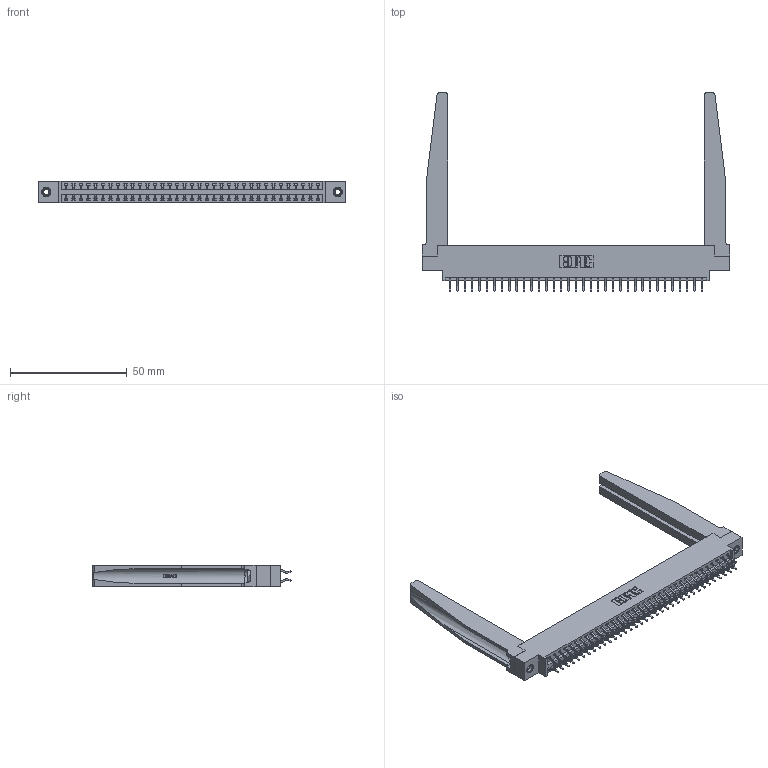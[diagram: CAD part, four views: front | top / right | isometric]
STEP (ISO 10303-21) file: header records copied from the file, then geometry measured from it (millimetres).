
FILE_DESCRIPTION (( 'STEP AP203' ), '1' );
FILE_NAME ('346-070-556-878.STEP', '2022-05-24T22:13:57', ( '' ), ( '' ), 'SwSTEP 2.0', 'SolidWorks 2020', '' );
FILE_SCHEMA (( 'CONFIG_CONTROL_DESIGN' ));
Length unit declared in the file: inch
Products named in the file (5): 345-250-001_345-250-001-102; 346-220-078_345-220-078; 346 Part_0.170 Offset - 0.156 Dia-TH; 346-070-556-878; 345-292-001_556 Tail
Assembly tree (75 placements, depth 2):
  346-070-556-878
    346 Part_0.170 Offset - 0.156 Dia-TH
    345-292-001_556 Tail  x70
    346-220-078_345-220-078  x2
    345-250-001_345-250-001-102  x2
Bounding box: 131.7 x 84.84 x 9.4 mm (x, y, z)
Volume: 19521.3 mm3; surface area: 23913.3 mm2
Topology: 75 solids, 75 shells, 4434 faces, 13095 edges, 8626 vertices
Faces by surface type: plane 2966, cylinder 1416, bspline 36, cone 12, torus 4
Entity records: 29300 total; most frequent: CARTESIAN_POINT 5797, ORIENTED_EDGE 4606, DIRECTION 4133, EDGE_CURVE 2303, VECTOR 1929, LINE 1929, VERTEX_POINT 1528, AXIS2_PLACEMENT_3D 1102
